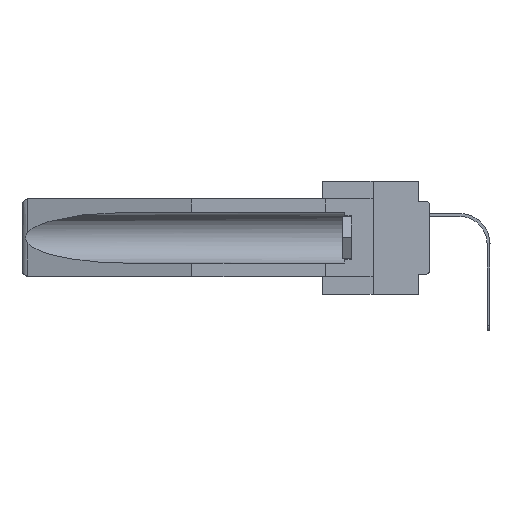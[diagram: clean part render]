
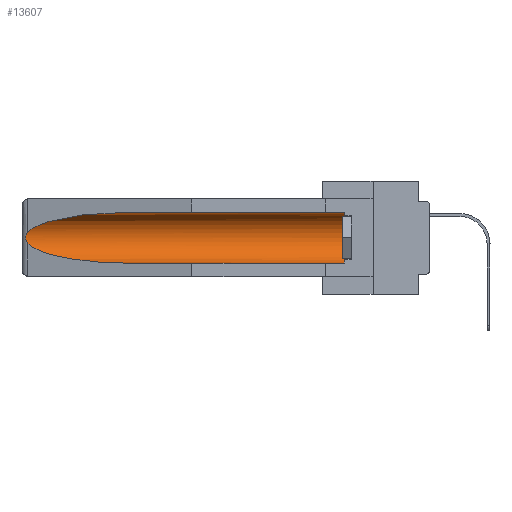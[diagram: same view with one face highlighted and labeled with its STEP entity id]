
A CAD part, left-side view. The second image highlights one B-rep face of the part: STEP entity #13607.
In plain terms, the highlighted cylindrical face has radius 2.857 mm (diameter 5.715 mm), a partial arc.
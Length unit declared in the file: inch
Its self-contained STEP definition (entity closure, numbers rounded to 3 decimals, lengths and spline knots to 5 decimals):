
#648 = VERTEX_POINT ( 'NONE', #29157 ) ;
#1115 = EDGE_CURVE ( 'NONE', #31337, #5821, #5752, .T. ) ;
#1961 = CARTESIAN_POINT ( 'NONE',  ( 0.26597, 1.5296, -0.19026 ) ) ;
#2759 = CARTESIAN_POINT ( 'NONE',  ( 0.155, 1.07973, -0.284 ) ) ;
#2841 = CYLINDRICAL_SURFACE ( 'NONE', #6662, 0.1125 ) ;
#3336 = ORIENTED_EDGE ( 'NONE', *, *, #32643, .T. ) ;
#3838 = CARTESIAN_POINT ( 'NONE',  ( 0.25451, 1.48313, -0.24835 ) ) ;
#4055 = EDGE_CURVE ( 'NONE', #648, #31337, #6121, .T. ) ;
#4690 = VECTOR ( 'NONE', #26266, 39.37008 ) ;
#5288 = LINE ( 'NONE', #28831, #4690 ) ;
#5372 = FACE_OUTER_BOUND ( 'NONE', #17603, .T. ) ;
#5752 =( BOUNDED_CURVE ( )  B_SPLINE_CURVE ( 3, ( #16873, #3838, #19247, #32266 ),
 .UNSPECIFIED., .F., .T. ) 
 B_SPLINE_CURVE_WITH_KNOTS ( ( 4, 4 ),
 ( 0.1948, 1.5708 ),
 .UNSPECIFIED. ) 
 CURVE ( )  GEOMETRIC_REPRESENTATION_ITEM ( )  RATIONAL_B_SPLINE_CURVE ( ( 1., 0.848, 0.848, 1. ) ) 
 REPRESENTATION_ITEM ( '' )  );
#5821 = VERTEX_POINT ( 'NONE', #2759 ) ;
#6121 = B_SPLINE_CURVE_WITH_KNOTS ( 'NONE', 3,
 ( #21940, #25145, #22435, #22114, #9728, #32763, #27856, #9560, #1961, #6541 ),
 .UNSPECIFIED., .F., .F.,
 ( 4, 2, 2, 2, 4 ),
 ( 0., 0.00029, 0.00058, 0.00087, 0.00117 ),
 .UNSPECIFIED. ) ;
#6541 = CARTESIAN_POINT ( 'NONE',  ( 0.26537, 1.52718, -0.19328 ) ) ;
#6662 = AXIS2_PLACEMENT_3D ( 'NONE', #25853, #11103, #8398 ) ;
#6947 = CARTESIAN_POINT ( 'NONE',  ( 0.155, 1.07973, -0.059 ) ) ;
#7480 = VECTOR ( 'NONE', #16893, 39.37008 ) ;
#7993 = ORIENTED_EDGE ( 'NONE', *, *, #4055, .T. ) ;
#8398 = DIRECTION ( 'NONE',  ( 0., 0., 1. ) ) ;
#9082 = LINE ( 'NONE', #9412, #7480 ) ;
#9412 = CARTESIAN_POINT ( 'NONE',  ( 0.155, -0.30754, -0.059 ) ) ;
#9560 = CARTESIAN_POINT ( 'NONE',  ( 0.26655, 1.53094, -0.18657 ) ) ;
#9644 = CARTESIAN_POINT ( 'NONE',  ( 0.26537, 1.52718, -0.14972 ) ) ;
#9728 = CARTESIAN_POINT ( 'NONE',  ( 0.2675, 1.53308, -0.16763 ) ) ;
#11103 = DIRECTION ( 'NONE',  ( 0., 1., 0. ) ) ;
#11188 = CARTESIAN_POINT ( 'NONE',  ( 0.155, 0.126, -0.059 ) ) ;
#12673 = CARTESIAN_POINT ( 'NONE',  ( 0.21114, 1.30732, -0.059 ) ) ;
#13388 = AXIS2_PLACEMENT_3D ( 'NONE', #27794, #22701, #33023 ) ;
#13607 = ADVANCED_FACE ( 'NONE', ( #5372 ), #2841, .F. ) ;
#15462 = EDGE_CURVE ( 'NONE', #18679, #5821, #5288, .T. ) ;
#15938 =( BOUNDED_CURVE ( )  B_SPLINE_CURVE ( 3, ( #6947, #12673, #20502, #9644 ),
 .UNSPECIFIED., .F., .T. ) 
 B_SPLINE_CURVE_WITH_KNOTS ( ( 4, 4 ),
 ( 4.71239, 6.08839 ),
 .UNSPECIFIED. ) 
 CURVE ( )  GEOMETRIC_REPRESENTATION_ITEM ( )  RATIONAL_B_SPLINE_CURVE ( ( 1., 0.848, 0.848, 1. ) ) 
 REPRESENTATION_ITEM ( '' )  );
#16873 = CARTESIAN_POINT ( 'NONE',  ( 0.26537, 1.52718, -0.19328 ) ) ;
#16893 = DIRECTION ( 'NONE',  ( 0., 1., 0. ) ) ;
#16954 = VERTEX_POINT ( 'NONE', #22577 ) ;
#17603 = EDGE_LOOP ( 'NONE', ( #18626, #7993, #26619, #30307, #22348, #3336 ) ) ;
#18626 = ORIENTED_EDGE ( 'NONE', *, *, #21650, .T. ) ;
#18679 = VERTEX_POINT ( 'NONE', #20313 ) ;
#19247 = CARTESIAN_POINT ( 'NONE',  ( 0.21114, 1.30732, -0.284 ) ) ;
#20313 = CARTESIAN_POINT ( 'NONE',  ( 0.155, 0.126, -0.284 ) ) ;
#20502 = CARTESIAN_POINT ( 'NONE',  ( 0.25451, 1.48313, -0.09465 ) ) ;
#21650 = EDGE_CURVE ( 'NONE', #16954, #648, #15938, .T. ) ;
#21940 = CARTESIAN_POINT ( 'NONE',  ( 0.26537, 1.52718, -0.14972 ) ) ;
#22114 = CARTESIAN_POINT ( 'NONE',  ( 0.2673, 1.5327, -0.16383 ) ) ;
#22348 = ORIENTED_EDGE ( 'NONE', *, *, #31893, .T. ) ;
#22435 = CARTESIAN_POINT ( 'NONE',  ( 0.26654, 1.53092, -0.15636 ) ) ;
#22577 = CARTESIAN_POINT ( 'NONE',  ( 0.155, 1.07973, -0.059 ) ) ;
#22701 = DIRECTION ( 'NONE',  ( 0., -1., 0. ) ) ;
#25087 = VERTEX_POINT ( 'NONE', #11188 ) ;
#25145 = CARTESIAN_POINT ( 'NONE',  ( 0.26597, 1.52961, -0.15275 ) ) ;
#25853 = CARTESIAN_POINT ( 'NONE',  ( 0.155, -0.30754, -0.1715 ) ) ;
#26266 = DIRECTION ( 'NONE',  ( 0., 1., 0. ) ) ;
#26619 = ORIENTED_EDGE ( 'NONE', *, *, #1115, .T. ) ;
#27664 = CARTESIAN_POINT ( 'NONE',  ( 0.26537, 1.52718, -0.19328 ) ) ;
#27794 = CARTESIAN_POINT ( 'NONE',  ( 0.155, 0.126, -0.1715 ) ) ;
#27856 = CARTESIAN_POINT ( 'NONE',  ( 0.2673, 1.53269, -0.17917 ) ) ;
#27978 = CIRCLE ( 'NONE', #13388, 0.1125 ) ;
#28831 = CARTESIAN_POINT ( 'NONE',  ( 0.155, -0.30754, -0.284 ) ) ;
#29157 = CARTESIAN_POINT ( 'NONE',  ( 0.26537, 1.52718, -0.14972 ) ) ;
#30307 = ORIENTED_EDGE ( 'NONE', *, *, #15462, .F. ) ;
#31337 = VERTEX_POINT ( 'NONE', #27664 ) ;
#31893 = EDGE_CURVE ( 'NONE', #18679, #25087, #27978, .T. ) ;
#32266 = CARTESIAN_POINT ( 'NONE',  ( 0.155, 1.07973, -0.284 ) ) ;
#32643 = EDGE_CURVE ( 'NONE', #25087, #16954, #9082, .T. ) ;
#32763 = CARTESIAN_POINT ( 'NONE',  ( 0.2675, 1.53308, -0.17534 ) ) ;
#33023 = DIRECTION ( 'NONE',  ( 0., 0., 1. ) ) ;
